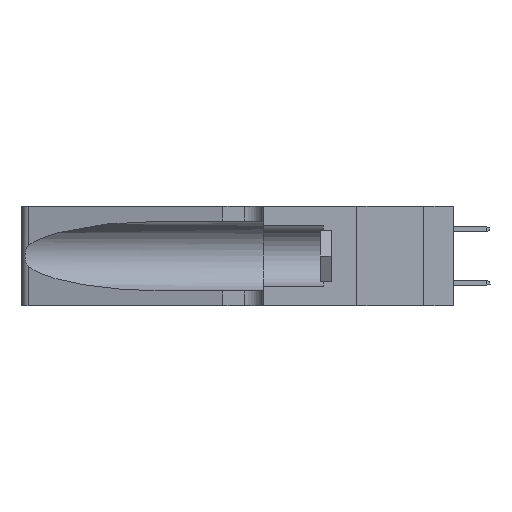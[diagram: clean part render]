
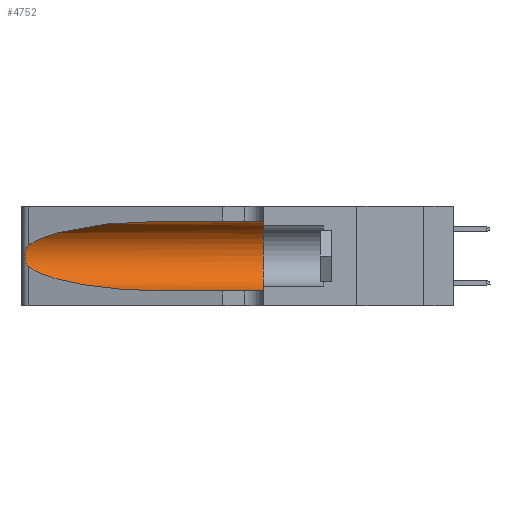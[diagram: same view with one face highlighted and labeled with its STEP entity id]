
A CAD part, left-side view. The second image highlights one B-rep face of the part: STEP entity #4752.
In plain terms, the highlighted cylindrical face has radius 3.308 mm (diameter 6.617 mm), a partial arc.
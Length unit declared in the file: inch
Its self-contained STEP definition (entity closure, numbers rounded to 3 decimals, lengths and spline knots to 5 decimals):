
#104 = CARTESIAN_POINT ( 'NONE',  ( 0.25555, 1.22994, 0.2215 ) ) ;
#538 = EDGE_CURVE ( 'NONE', #21547, #30621, #22754, .T. ) ;
#1835 = ORIENTED_EDGE ( 'NONE', *, *, #538, .F. ) ;
#2311 = CARTESIAN_POINT ( 'NONE',  ( 0.25639, 1.23184, 0.21858 ) ) ;
#2870 = EDGE_CURVE ( 'NONE', #21547, #17119, #6847, .T. ) ;
#3511 = B_SPLINE_CURVE_WITH_KNOTS ( 'NONE', 3,
 ( #23691, #104, #2311, #11859, #18713, #23840, #9665, #28178, #28637, #23534, #21661, #6710, #7329, #16228 ),
 .UNSPECIFIED., .F., .F.,
 ( 4, 2, 2, 2, 2, 2, 4 ),
 ( 0., 0.00027, 0.00053, 0.00107, 0.0016, 0.00187, 0.00214 ),
 .UNSPECIFIED. ) ;
#3765 = CARTESIAN_POINT ( 'NONE',  ( 0.1305, 0.35, 0.185 ) ) ;
#3953 = VERTEX_POINT ( 'NONE', #21695 ) ;
#4227 = DIRECTION ( 'NONE',  ( 0., -1., 0. ) ) ;
#4752 = ADVANCED_FACE ( 'NONE', ( #9630 ), #6670, .F. ) ;
#6670 = CYLINDRICAL_SURFACE ( 'NONE', #29054, 0.13025 ) ;
#6710 = CARTESIAN_POINT ( 'NONE',  ( 0.25639, 1.23186, 0.15144 ) ) ;
#6847 =( BOUNDED_CURVE ( )  B_SPLINE_CURVE ( 3, ( #20497, #11462, #15668, #25462 ),
 .UNSPECIFIED., .F., .T. ) 
 B_SPLINE_CURVE_WITH_KNOTS ( ( 4, 4 ),
 ( 1.5708, 2.84003 ),
 .UNSPECIFIED. ) 
 CURVE ( )  GEOMETRIC_REPRESENTATION_ITEM ( )  RATIONAL_B_SPLINE_CURVE ( ( 1., 0.87, 0.87, 1. ) ) 
 REPRESENTATION_ITEM ( '' )  );
#7122 = ORIENTED_EDGE ( 'NONE', *, *, #2870, .T. ) ;
#7329 = CARTESIAN_POINT ( 'NONE',  ( 0.25555, 1.22993, 0.14849 ) ) ;
#7939 = DIRECTION ( 'NONE',  ( 0., -1., 0. ) ) ;
#8119 = EDGE_CURVE ( 'NONE', #30621, #28254, #12822, .T. ) ;
#8149 = DIRECTION ( 'NONE',  ( 0., 1., 0. ) ) ;
#8409 = ORIENTED_EDGE ( 'NONE', *, *, #27544, .T. ) ;
#9435 = VECTOR ( 'NONE', #7939, 39.37008 ) ;
#9480 = CARTESIAN_POINT ( 'NONE',  ( 0.1305, 1.61858, 0.185 ) ) ;
#9630 = FACE_OUTER_BOUND ( 'NONE', #21110, .T. ) ;
#9665 = CARTESIAN_POINT ( 'NONE',  ( 0.26075, 1.23896, 0.19203 ) ) ;
#9728 = CARTESIAN_POINT ( 'NONE',  ( 0.1305, 0.35, 0.05475 ) ) ;
#10597 = CARTESIAN_POINT ( 'NONE',  ( 0.1305, 1.61858, 0.31525 ) ) ;
#11180 = CARTESIAN_POINT ( 'NONE',  ( 0.18966, 0.96281, 0.05475 ) ) ;
#11389 = ORIENTED_EDGE ( 'NONE', *, *, #14389, .T. ) ;
#11462 = CARTESIAN_POINT ( 'NONE',  ( 0.18966, 0.96281, 0.31525 ) ) ;
#11859 = CARTESIAN_POINT ( 'NONE',  ( 0.25787, 1.23484, 0.2124 ) ) ;
#12349 = EDGE_CURVE ( 'NONE', #21435, #28254, #27911, .T. ) ;
#12822 = CIRCLE ( 'NONE', #28702, 0.13025 ) ;
#14137 = CARTESIAN_POINT ( 'NONE',  ( 0.1305, 0.72297, 0.05475 ) ) ;
#14389 = EDGE_CURVE ( 'NONE', #17119, #3953, #3511, .T. ) ;
#15668 = CARTESIAN_POINT ( 'NONE',  ( 0.2373, 1.15595, 0.28018 ) ) ;
#16228 = CARTESIAN_POINT ( 'NONE',  ( 0.25487, 1.22718, 0.14631 ) ) ;
#16321 = CARTESIAN_POINT ( 'NONE',  ( 0.25487, 1.22718, 0.14631 ) ) ;
#16410 =( BOUNDED_CURVE ( )  B_SPLINE_CURVE ( 3, ( #16321, #21132, #11180, #14137 ),
 .UNSPECIFIED., .F., .F. ) 
 B_SPLINE_CURVE_WITH_KNOTS ( ( 4, 4 ),
 ( 3.44316, 4.71239 ),
 .UNSPECIFIED. ) 
 CURVE ( )  GEOMETRIC_REPRESENTATION_ITEM ( )  RATIONAL_B_SPLINE_CURVE ( ( 1., 0.87, 0.87, 1. ) ) 
 REPRESENTATION_ITEM ( '' )  );
#17119 = VERTEX_POINT ( 'NONE', #17964 ) ;
#17890 = ORIENTED_EDGE ( 'NONE', *, *, #8119, .F. ) ;
#17912 = VECTOR ( 'NONE', #4227, 39.37008 ) ;
#17964 = CARTESIAN_POINT ( 'NONE',  ( 0.25487, 1.22718, 0.22369 ) ) ;
#18414 = ORIENTED_EDGE ( 'NONE', *, *, #12349, .T. ) ;
#18713 = CARTESIAN_POINT ( 'NONE',  ( 0.25854, 1.2359, 0.20912 ) ) ;
#18982 = DIRECTION ( 'NONE',  ( 0., 0., -1. ) ) ;
#20497 = CARTESIAN_POINT ( 'NONE',  ( 0.1305, 0.72297, 0.31525 ) ) ;
#20772 = CARTESIAN_POINT ( 'NONE',  ( 0.1305, 1.61858, 0.05475 ) ) ;
#21110 = EDGE_LOOP ( 'NONE', ( #7122, #11389, #8409, #18414, #17890, #1835 ) ) ;
#21132 = CARTESIAN_POINT ( 'NONE',  ( 0.2373, 1.15595, 0.08982 ) ) ;
#21309 = DIRECTION ( 'NONE',  ( 0., -1., 0. ) ) ;
#21435 = VERTEX_POINT ( 'NONE', #23670 ) ;
#21547 = VERTEX_POINT ( 'NONE', #26739 ) ;
#21585 = CARTESIAN_POINT ( 'NONE',  ( 0.1305, 0.35, 0.31525 ) ) ;
#21661 = CARTESIAN_POINT ( 'NONE',  ( 0.25789, 1.23486, 0.15765 ) ) ;
#21695 = CARTESIAN_POINT ( 'NONE',  ( 0.25487, 1.22718, 0.14631 ) ) ;
#22754 = LINE ( 'NONE', #10597, #9435 ) ;
#23534 = CARTESIAN_POINT ( 'NONE',  ( 0.25856, 1.23593, 0.16098 ) ) ;
#23670 = CARTESIAN_POINT ( 'NONE',  ( 0.1305, 0.72297, 0.05475 ) ) ;
#23691 = CARTESIAN_POINT ( 'NONE',  ( 0.25487, 1.22718, 0.22369 ) ) ;
#23840 = CARTESIAN_POINT ( 'NONE',  ( 0.26018, 1.23835, 0.19895 ) ) ;
#24819 = DIRECTION ( 'NONE',  ( 0., 0., 1. ) ) ;
#25462 = CARTESIAN_POINT ( 'NONE',  ( 0.25487, 1.22718, 0.22369 ) ) ;
#26739 = CARTESIAN_POINT ( 'NONE',  ( 0.1305, 0.72297, 0.31525 ) ) ;
#27544 = EDGE_CURVE ( 'NONE', #3953, #21435, #16410, .T. ) ;
#27911 = LINE ( 'NONE', #20772, #17912 ) ;
#28178 = CARTESIAN_POINT ( 'NONE',  ( 0.26075, 1.23896, 0.178 ) ) ;
#28254 = VERTEX_POINT ( 'NONE', #9728 ) ;
#28637 = CARTESIAN_POINT ( 'NONE',  ( 0.26017, 1.23833, 0.17102 ) ) ;
#28702 = AXIS2_PLACEMENT_3D ( 'NONE', #3765, #8149, #24819 ) ;
#29054 = AXIS2_PLACEMENT_3D ( 'NONE', #9480, #21309, #18982 ) ;
#30621 = VERTEX_POINT ( 'NONE', #21585 ) ;
